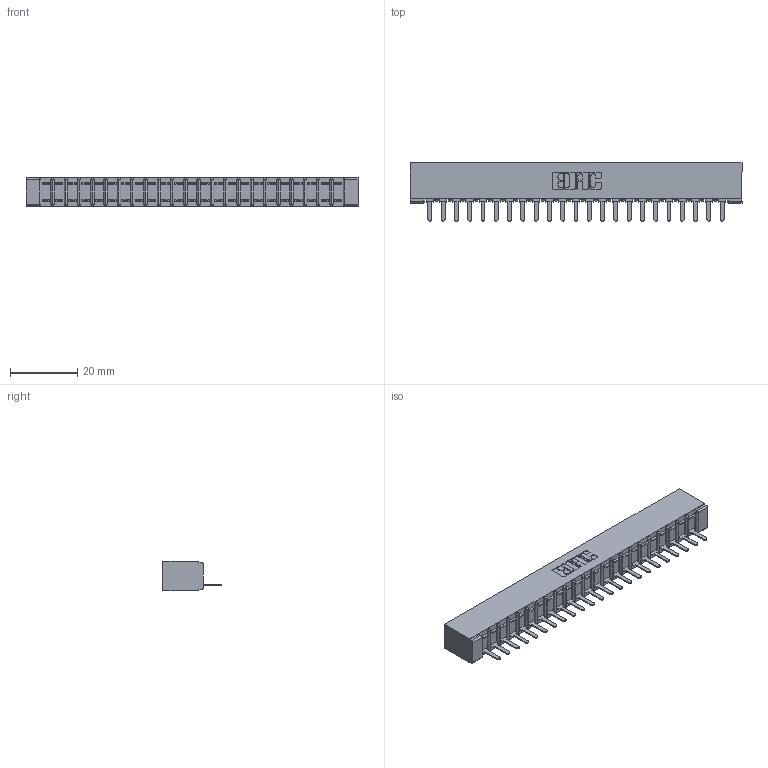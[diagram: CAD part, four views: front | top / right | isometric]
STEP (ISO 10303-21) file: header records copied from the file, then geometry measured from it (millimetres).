
FILE_DESCRIPTION (( 'STEP AP203' ), '1' );
FILE_NAME ('307-023-521-101.STEP', '2018-08-04T05:20:54', ( '' ), ( '' ), 'SwSTEP 2.0', 'SolidWorks 2016', '' );
FILE_SCHEMA (( 'CONFIG_CONTROL_DESIGN' ));
Length unit declared in the file: inch
Products named in the file (3): 307 Part_No Mounting Lugs; 307-290-002_521; 307-023-521-101
Assembly tree (24 placements, depth 2):
  307-023-521-101
    307 Part_No Mounting Lugs
    307-290-002_521  x23
Bounding box: 99.01 x 17.42 x 8.71 mm (x, y, z)
Volume: 6780.6 mm3; surface area: 12909.3 mm2
Topology: 24 solids, 24 shells, 1836 faces, 5635 edges, 3690 vertices
Faces by surface type: plane 1101, cylinder 687, sphere 48
Entity records: 22500 total; most frequent: CARTESIAN_POINT 3792, ORIENTED_EDGE 3782, DIRECTION 3691, EDGE_CURVE 1891, LINE 1441, VECTOR 1441, VERTEX_POINT 1226, AXIS2_PLACEMENT_3D 1125
